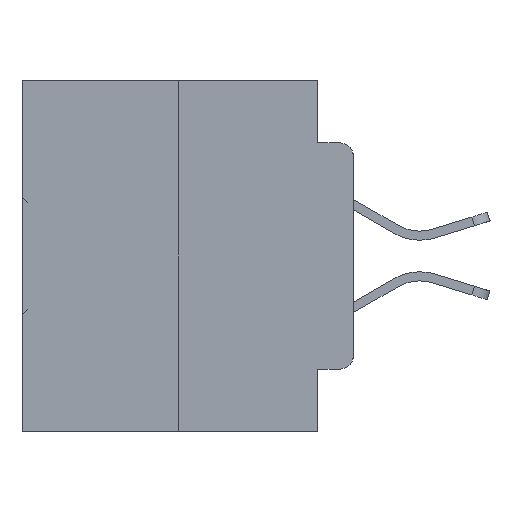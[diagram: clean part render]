
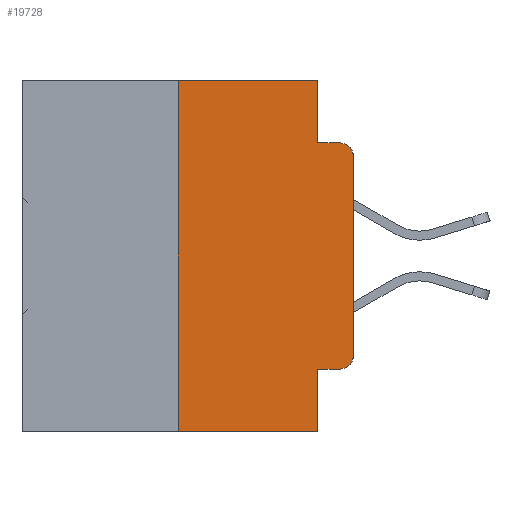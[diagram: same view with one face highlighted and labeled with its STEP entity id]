
A CAD part, left-side view. The second image highlights one B-rep face of the part: STEP entity #19728.
In plain terms, the highlighted planar face has unit normal (-1, 0, 0).
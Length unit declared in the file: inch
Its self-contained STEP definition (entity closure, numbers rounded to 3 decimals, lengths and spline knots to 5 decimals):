
#253 = CARTESIAN_POINT ( 'NONE',  ( 0., 0.051, -0.5 ) ) ;
#507 = AXIS2_PLACEMENT_3D ( 'NONE', #32085, #12681, #26932 ) ;
#1577 = DIRECTION ( 'NONE',  ( 0., 0., -1. ) ) ;
#2056 = LINE ( 'NONE', #18928, #24914 ) ;
#2327 = CARTESIAN_POINT ( 'NONE',  ( 0., 0.051, -0.4115 ) ) ;
#2458 = VERTEX_POINT ( 'NONE', #19958 ) ;
#2802 = DIRECTION ( 'NONE',  ( 0., -1., 0. ) ) ;
#3001 = DIRECTION ( 'NONE',  ( 0., 0., 1. ) ) ;
#3080 = ORIENTED_EDGE ( 'NONE', *, *, #24557, .T. ) ;
#3141 = VERTEX_POINT ( 'NONE', #4073 ) ;
#3234 = CARTESIAN_POINT ( 'NONE',  ( 0., 0., -0.3915 ) ) ;
#3304 = CARTESIAN_POINT ( 'NONE',  ( 0., 0.051, 0. ) ) ;
#4073 = CARTESIAN_POINT ( 'NONE',  ( 0., 0.02, -0.4115 ) ) ;
#4369 = CARTESIAN_POINT ( 'NONE',  ( 0., 0.25, 0. ) ) ;
#4616 = DIRECTION ( 'NONE',  ( 0., 0., 1. ) ) ;
#5286 = VERTEX_POINT ( 'NONE', #17986 ) ;
#6653 = VECTOR ( 'NONE', #22919, 39.37008 ) ;
#6910 = PLANE ( 'NONE',  #507 ) ;
#7752 = EDGE_CURVE ( 'NONE', #2458, #5286, #14145, .T. ) ;
#8145 = LINE ( 'NONE', #9153, #26562 ) ;
#8318 = DIRECTION ( 'NONE',  ( 0., -1., 0. ) ) ;
#8594 = VECTOR ( 'NONE', #12607, 39.37008 ) ;
#8607 = DIRECTION ( 'NONE',  ( 0., 0., -1. ) ) ;
#8683 = CIRCLE ( 'NONE', #9675, 0.02 ) ;
#8745 = CARTESIAN_POINT ( 'NONE',  ( 0., 0., 0. ) ) ;
#8765 = CARTESIAN_POINT ( 'NONE',  ( 0., 0., -0.1085 ) ) ;
#9153 = CARTESIAN_POINT ( 'NONE',  ( 0., 0.051, 0. ) ) ;
#9675 = AXIS2_PLACEMENT_3D ( 'NONE', #14032, #19799, #8607 ) ;
#9942 = CARTESIAN_POINT ( 'NONE',  ( 0., 0.02, -0.0885 ) ) ;
#11396 = AXIS2_PLACEMENT_3D ( 'NONE', #11673, #17367, #19943 ) ;
#11448 = EDGE_CURVE ( 'NONE', #5286, #32267, #34966, .T. ) ;
#11673 = CARTESIAN_POINT ( 'NONE',  ( 0., 0.02, -0.1085 ) ) ;
#11915 = ORIENTED_EDGE ( 'NONE', *, *, #11448, .F. ) ;
#11956 = EDGE_CURVE ( 'NONE', #32974, #32570, #8145, .T. ) ;
#12607 = DIRECTION ( 'NONE',  ( 0., -1., 0. ) ) ;
#12681 = DIRECTION ( 'NONE',  ( 1., 0., 0. ) ) ;
#13009 = LINE ( 'NONE', #8745, #32381 ) ;
#13273 = VECTOR ( 'NONE', #8318, 39.37008 ) ;
#14032 = CARTESIAN_POINT ( 'NONE',  ( 0., 0.02, -0.3915 ) ) ;
#14145 = LINE ( 'NONE', #3304, #6653 ) ;
#16108 = ORIENTED_EDGE ( 'NONE', *, *, #33832, .T. ) ;
#17367 = DIRECTION ( 'NONE',  ( -1., 0., 0. ) ) ;
#17630 = VECTOR ( 'NONE', #4616, 39.37008 ) ;
#17768 = VERTEX_POINT ( 'NONE', #3234 ) ;
#17986 = CARTESIAN_POINT ( 'NONE',  ( 0., 0.051, -0.0885 ) ) ;
#18054 = LINE ( 'NONE', #4369, #17630 ) ;
#18221 = EDGE_CURVE ( 'NONE', #27354, #2458, #34945, .T. ) ;
#18453 = ORIENTED_EDGE ( 'NONE', *, *, #7752, .F. ) ;
#18928 = CARTESIAN_POINT ( 'NONE',  ( 0., 0.473, -0.5 ) ) ;
#19375 = CARTESIAN_POINT ( 'NONE',  ( 0., 0.051, -0.0885 ) ) ;
#19550 = DIRECTION ( 'NONE',  ( 0., -1., 0. ) ) ;
#19728 = ADVANCED_FACE ( 'NONE', ( #33353 ), #6910, .F. ) ;
#19799 = DIRECTION ( 'NONE',  ( -1., 0., 0. ) ) ;
#19943 = DIRECTION ( 'NONE',  ( 0., 0., -1. ) ) ;
#19958 = CARTESIAN_POINT ( 'NONE',  ( 0., 0.051, 0. ) ) ;
#21555 = ORIENTED_EDGE ( 'NONE', *, *, #18221, .F. ) ;
#21744 = CARTESIAN_POINT ( 'NONE',  ( 0., 0.25, 0. ) ) ;
#21966 = CARTESIAN_POINT ( 'NONE',  ( 0., 0.051, -0.4115 ) ) ;
#22919 = DIRECTION ( 'NONE',  ( 0., 0., -1. ) ) ;
#23602 = VERTEX_POINT ( 'NONE', #27933 ) ;
#23737 = EDGE_CURVE ( 'NONE', #32974, #3141, #30462, .T. ) ;
#23767 = CIRCLE ( 'NONE', #11396, 0.02 ) ;
#24557 = EDGE_CURVE ( 'NONE', #30684, #32267, #23767, .T. ) ;
#24914 = VECTOR ( 'NONE', #19550, 39.37008 ) ;
#24954 = EDGE_CURVE ( 'NONE', #23602, #27354, #18054, .T. ) ;
#25619 = EDGE_LOOP ( 'NONE', ( #16108, #3080, #11915, #18453, #21555, #25684, #30978, #32880, #33114, #27893 ) ) ;
#25684 = ORIENTED_EDGE ( 'NONE', *, *, #24954, .F. ) ;
#26562 = VECTOR ( 'NONE', #1577, 39.37008 ) ;
#26594 = CARTESIAN_POINT ( 'NONE',  ( 0., 0.473, 0. ) ) ;
#26932 = DIRECTION ( 'NONE',  ( 0., 0., -1. ) ) ;
#27354 = VERTEX_POINT ( 'NONE', #21744 ) ;
#27893 = ORIENTED_EDGE ( 'NONE', *, *, #31198, .T. ) ;
#27933 = CARTESIAN_POINT ( 'NONE',  ( 0., 0.25, -0.5 ) ) ;
#29709 = VECTOR ( 'NONE', #2802, 39.37008 ) ;
#30462 = LINE ( 'NONE', #2327, #13273 ) ;
#30684 = VERTEX_POINT ( 'NONE', #8765 ) ;
#30978 = ORIENTED_EDGE ( 'NONE', *, *, #31728, .T. ) ;
#31198 = EDGE_CURVE ( 'NONE', #3141, #17768, #8683, .T. ) ;
#31728 = EDGE_CURVE ( 'NONE', #23602, #32570, #2056, .T. ) ;
#32085 = CARTESIAN_POINT ( 'NONE',  ( 0., 0.473, 0. ) ) ;
#32267 = VERTEX_POINT ( 'NONE', #9942 ) ;
#32381 = VECTOR ( 'NONE', #3001, 39.37008 ) ;
#32570 = VERTEX_POINT ( 'NONE', #253 ) ;
#32880 = ORIENTED_EDGE ( 'NONE', *, *, #11956, .F. ) ;
#32974 = VERTEX_POINT ( 'NONE', #21966 ) ;
#33114 = ORIENTED_EDGE ( 'NONE', *, *, #23737, .T. ) ;
#33353 = FACE_OUTER_BOUND ( 'NONE', #25619, .T. ) ;
#33832 = EDGE_CURVE ( 'NONE', #17768, #30684, #13009, .T. ) ;
#34945 = LINE ( 'NONE', #26594, #8594 ) ;
#34966 = LINE ( 'NONE', #19375, #29709 ) ;
